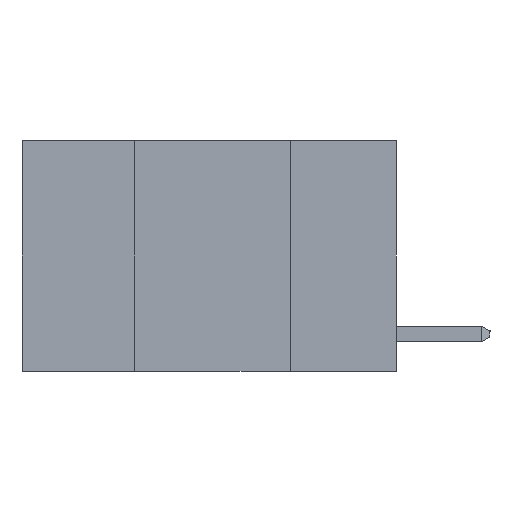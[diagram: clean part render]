
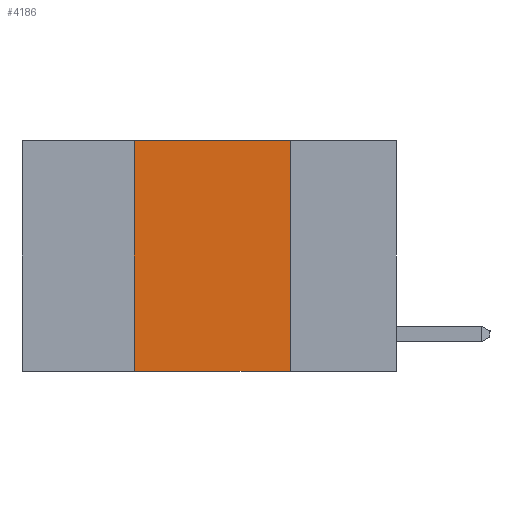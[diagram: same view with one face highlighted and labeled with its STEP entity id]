
A CAD part, left-side view. The second image highlights one B-rep face of the part: STEP entity #4186.
In plain terms, the highlighted planar face has unit normal (-1, 0, 0).
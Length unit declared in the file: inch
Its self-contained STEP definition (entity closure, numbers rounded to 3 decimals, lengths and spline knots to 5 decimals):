
#108 = VECTOR ( 'NONE', #6830, 39.37008 ) ;
#666 = LINE ( 'NONE', #8643, #7669 ) ;
#820 = CARTESIAN_POINT ( 'NONE',  ( 0., 0.42, 0. ) ) ;
#996 = CARTESIAN_POINT ( 'NONE',  ( 0., 0.6, -0.37 ) ) ;
#1019 = AXIS2_PLACEMENT_3D ( 'NONE', #10570, #10548, #10533 ) ;
#1029 = DIRECTION ( 'NONE',  ( 0., 0., 1. ) ) ;
#1060 = CARTESIAN_POINT ( 'NONE',  ( 0., 0.42, 0. ) ) ;
#1837 = ORIENTED_EDGE ( 'NONE', *, *, #10082, .F. ) ;
#1860 = EDGE_CURVE ( 'NONE', #6305, #14317, #666, .T. ) ;
#2170 = ORIENTED_EDGE ( 'NONE', *, *, #1860, .F. ) ;
#2658 = FACE_OUTER_BOUND ( 'NONE', #5668, .T. ) ;
#3657 = DIRECTION ( 'NONE',  ( 0., -1., 0. ) ) ;
#3761 = EDGE_CURVE ( 'NONE', #11182, #6305, #6608, .T. ) ;
#3912 = ORIENTED_EDGE ( 'NONE', *, *, #3761, .F. ) ;
#4186 = ADVANCED_FACE ( 'NONE', ( #2658 ), #10666, .F. ) ;
#5125 = ORIENTED_EDGE ( 'NONE', *, *, #5851, .T. ) ;
#5515 = CARTESIAN_POINT ( 'NONE',  ( 0., 0.17, 0. ) ) ;
#5668 = EDGE_LOOP ( 'NONE', ( #1837, #2170, #3912, #5125 ) ) ;
#5738 = VERTEX_POINT ( 'NONE', #14916 ) ;
#5851 = EDGE_CURVE ( 'NONE', #11182, #5738, #9182, .T. ) ;
#5991 = CARTESIAN_POINT ( 'NONE',  ( 0., 0.42, -0.37 ) ) ;
#6305 = VERTEX_POINT ( 'NONE', #820 ) ;
#6608 = LINE ( 'NONE', #1060, #9634 ) ;
#6830 = DIRECTION ( 'NONE',  ( 0., 0., -1. ) ) ;
#7127 = LINE ( 'NONE', #5515, #108 ) ;
#7397 = CARTESIAN_POINT ( 'NONE',  ( 0., 0.17, 0. ) ) ;
#7669 = VECTOR ( 'NONE', #11853, 39.37008 ) ;
#8643 = CARTESIAN_POINT ( 'NONE',  ( 0., 0.6, 0. ) ) ;
#9182 = LINE ( 'NONE', #996, #11353 ) ;
#9634 = VECTOR ( 'NONE', #1029, 39.37008 ) ;
#10082 = EDGE_CURVE ( 'NONE', #14317, #5738, #7127, .T. ) ;
#10533 = DIRECTION ( 'NONE',  ( 0., 0., -1. ) ) ;
#10548 = DIRECTION ( 'NONE',  ( 1., 0., 0. ) ) ;
#10570 = CARTESIAN_POINT ( 'NONE',  ( 0., 0.6, 0. ) ) ;
#10666 = PLANE ( 'NONE',  #1019 ) ;
#11182 = VERTEX_POINT ( 'NONE', #5991 ) ;
#11353 = VECTOR ( 'NONE', #3657, 39.37008 ) ;
#11853 = DIRECTION ( 'NONE',  ( 0., -1., 0. ) ) ;
#14317 = VERTEX_POINT ( 'NONE', #7397 ) ;
#14916 = CARTESIAN_POINT ( 'NONE',  ( 0., 0.17, -0.37 ) ) ;
